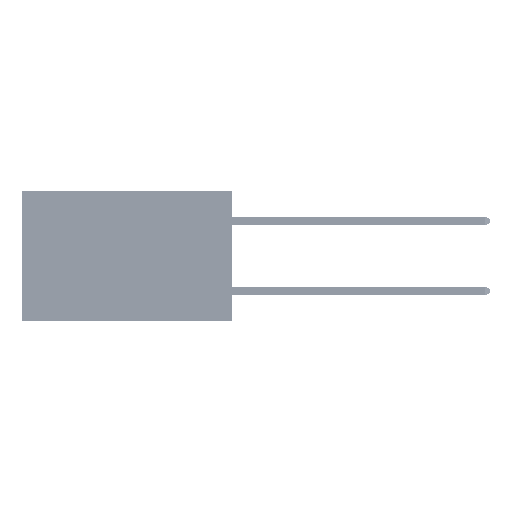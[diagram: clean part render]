
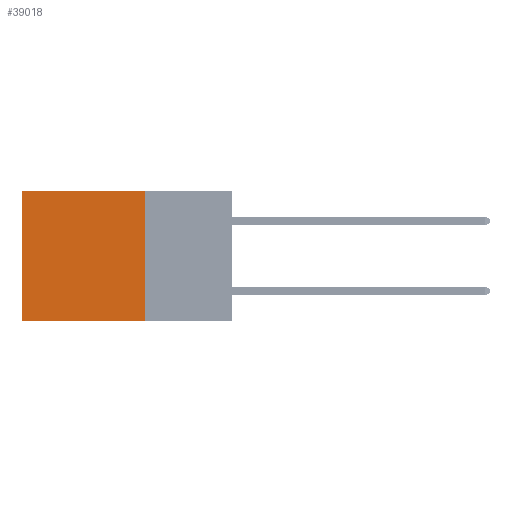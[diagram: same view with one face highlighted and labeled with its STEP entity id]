
A CAD part, left-side view. The second image highlights one B-rep face of the part: STEP entity #39018.
In plain terms, the highlighted planar face has unit normal (-1, 0, 0).
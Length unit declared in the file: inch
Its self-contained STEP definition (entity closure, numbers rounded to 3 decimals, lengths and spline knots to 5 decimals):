
#1268 = DIRECTION ( 'NONE',  ( 0., 0., -1. ) ) ;
#1662 = DIRECTION ( 'NONE',  ( 1., 0., 0. ) ) ;
#3037 = VERTEX_POINT ( 'NONE', #15309 ) ;
#3533 = ORIENTED_EDGE ( 'NONE', *, *, #19086, .T. ) ;
#4063 = EDGE_CURVE ( 'NONE', #3037, #17054, #47640, .T. ) ;
#4207 = CARTESIAN_POINT ( 'NONE',  ( 0.2875, 0.25, 0. ) ) ;
#5415 = DIRECTION ( 'NONE',  ( 0., 0., -1. ) ) ;
#6243 = VECTOR ( 'NONE', #24520, 39.37008 ) ;
#7502 = CARTESIAN_POINT ( 'NONE',  ( 0.2875, 0.6, -0.37 ) ) ;
#10596 = VECTOR ( 'NONE', #1268, 39.37008 ) ;
#11060 = ORIENTED_EDGE ( 'NONE', *, *, #40166, .F. ) ;
#13215 = CARTESIAN_POINT ( 'NONE',  ( 0.2875, 0.6, 0. ) ) ;
#15309 = CARTESIAN_POINT ( 'NONE',  ( 0.2875, 0.25, 0. ) ) ;
#15884 = CARTESIAN_POINT ( 'NONE',  ( 0.2875, 0.25, 0. ) ) ;
#17054 = VERTEX_POINT ( 'NONE', #23294 ) ;
#18006 = EDGE_CURVE ( 'NONE', #33991, #43794, #33252, .T. ) ;
#18638 = VECTOR ( 'NONE', #27143, 39.37008 ) ;
#19086 = EDGE_CURVE ( 'NONE', #3037, #33991, #23273, .T. ) ;
#22178 = AXIS2_PLACEMENT_3D ( 'NONE', #46618, #1662, #5415 ) ;
#23273 = LINE ( 'NONE', #15884, #36103 ) ;
#23294 = CARTESIAN_POINT ( 'NONE',  ( 0.2875, 0.25, -0.37 ) ) ;
#24520 = DIRECTION ( 'NONE',  ( 0., 0., -1. ) ) ;
#26732 = DIRECTION ( 'NONE',  ( 0., 1., 0. ) ) ;
#27143 = DIRECTION ( 'NONE',  ( 0., 1., 0. ) ) ;
#28062 = PLANE ( 'NONE',  #22178 ) ;
#33052 = EDGE_LOOP ( 'NONE', ( #37256, #11060, #40865, #3533 ) ) ;
#33252 = LINE ( 'NONE', #13215, #6243 ) ;
#33991 = VERTEX_POINT ( 'NONE', #45507 ) ;
#36103 = VECTOR ( 'NONE', #26732, 39.37008 ) ;
#37256 = ORIENTED_EDGE ( 'NONE', *, *, #18006, .T. ) ;
#39018 = ADVANCED_FACE ( 'NONE', ( #48137 ), #28062, .F. ) ;
#40166 = EDGE_CURVE ( 'NONE', #17054, #43794, #44579, .T. ) ;
#40865 = ORIENTED_EDGE ( 'NONE', *, *, #4063, .F. ) ;
#42046 = CARTESIAN_POINT ( 'NONE',  ( 0.2875, 0.25, -0.37 ) ) ;
#43794 = VERTEX_POINT ( 'NONE', #7502 ) ;
#44579 = LINE ( 'NONE', #42046, #18638 ) ;
#45507 = CARTESIAN_POINT ( 'NONE',  ( 0.2875, 0.6, 0. ) ) ;
#46618 = CARTESIAN_POINT ( 'NONE',  ( 0.2875, 0.25, 0. ) ) ;
#47640 = LINE ( 'NONE', #4207, #10596 ) ;
#48137 = FACE_OUTER_BOUND ( 'NONE', #33052, .T. ) ;
